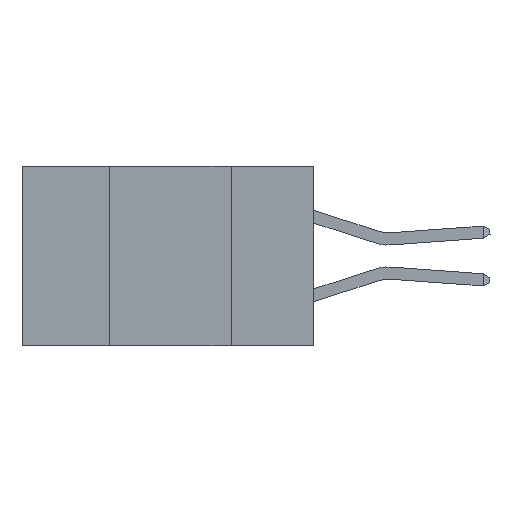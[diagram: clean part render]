
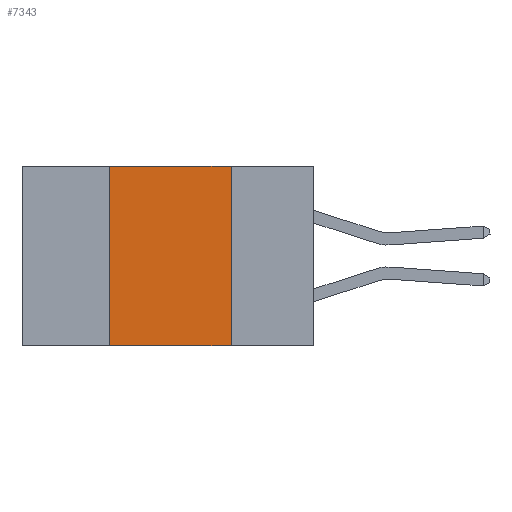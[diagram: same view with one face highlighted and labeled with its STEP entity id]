
A CAD part, left-side view. The second image highlights one B-rep face of the part: STEP entity #7343.
In plain terms, the highlighted planar face has unit normal (-1, 0, 0).
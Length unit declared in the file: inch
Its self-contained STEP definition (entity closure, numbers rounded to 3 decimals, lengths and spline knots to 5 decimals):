
#462 = DIRECTION ( 'NONE',  ( 0., -1., 0. ) ) ;
#520 = ORIENTED_EDGE ( 'NONE', *, *, #4375, .F. ) ;
#1060 = LINE ( 'NONE', #10592, #6184 ) ;
#1151 = CARTESIAN_POINT ( 'NONE',  ( 0., 0.17, -0.37 ) ) ;
#1357 = PLANE ( 'NONE',  #1946 ) ;
#1487 = FACE_OUTER_BOUND ( 'NONE', #7512, .T. ) ;
#1946 = AXIS2_PLACEMENT_3D ( 'NONE', #9669, #11905, #2587 ) ;
#2122 = VECTOR ( 'NONE', #462, 39.37008 ) ;
#2587 = DIRECTION ( 'NONE',  ( 0., 0., -1. ) ) ;
#2721 = CARTESIAN_POINT ( 'NONE',  ( 0., 0.6, 0. ) ) ;
#3265 = VERTEX_POINT ( 'NONE', #10940 ) ;
#3851 = VECTOR ( 'NONE', #12517, 39.37008 ) ;
#3866 = ORIENTED_EDGE ( 'NONE', *, *, #9765, .F. ) ;
#4148 = LINE ( 'NONE', #4415, #3851 ) ;
#4183 = CARTESIAN_POINT ( 'NONE',  ( 0., 0.17, 0. ) ) ;
#4375 = EDGE_CURVE ( 'NONE', #9207, #13459, #4148, .T. ) ;
#4415 = CARTESIAN_POINT ( 'NONE',  ( 0., 0.17, 0. ) ) ;
#4614 = EDGE_CURVE ( 'NONE', #3265, #13459, #12987, .T. ) ;
#6184 = VECTOR ( 'NONE', #8210, 39.37008 ) ;
#6656 = CARTESIAN_POINT ( 'NONE',  ( 0., 0.6, -0.37 ) ) ;
#6919 = DIRECTION ( 'NONE',  ( 0., -1., 0. ) ) ;
#7005 = VERTEX_POINT ( 'NONE', #13276 ) ;
#7127 = LINE ( 'NONE', #2721, #11615 ) ;
#7343 = ADVANCED_FACE ( 'NONE', ( #1487 ), #1357, .F. ) ;
#7512 = EDGE_LOOP ( 'NONE', ( #520, #3866, #11728, #8034 ) ) ;
#8034 = ORIENTED_EDGE ( 'NONE', *, *, #4614, .T. ) ;
#8210 = DIRECTION ( 'NONE',  ( 0., 0., 1. ) ) ;
#9207 = VERTEX_POINT ( 'NONE', #4183 ) ;
#9669 = CARTESIAN_POINT ( 'NONE',  ( 0., 0.6, 0. ) ) ;
#9765 = EDGE_CURVE ( 'NONE', #7005, #9207, #7127, .T. ) ;
#9858 = EDGE_CURVE ( 'NONE', #3265, #7005, #1060, .T. ) ;
#10592 = CARTESIAN_POINT ( 'NONE',  ( 0., 0.42, 0. ) ) ;
#10940 = CARTESIAN_POINT ( 'NONE',  ( 0., 0.42, -0.37 ) ) ;
#11615 = VECTOR ( 'NONE', #6919, 39.37008 ) ;
#11728 = ORIENTED_EDGE ( 'NONE', *, *, #9858, .F. ) ;
#11905 = DIRECTION ( 'NONE',  ( 1., 0., 0. ) ) ;
#12517 = DIRECTION ( 'NONE',  ( 0., 0., -1. ) ) ;
#12987 = LINE ( 'NONE', #6656, #2122 ) ;
#13276 = CARTESIAN_POINT ( 'NONE',  ( 0., 0.42, 0. ) ) ;
#13459 = VERTEX_POINT ( 'NONE', #1151 ) ;
